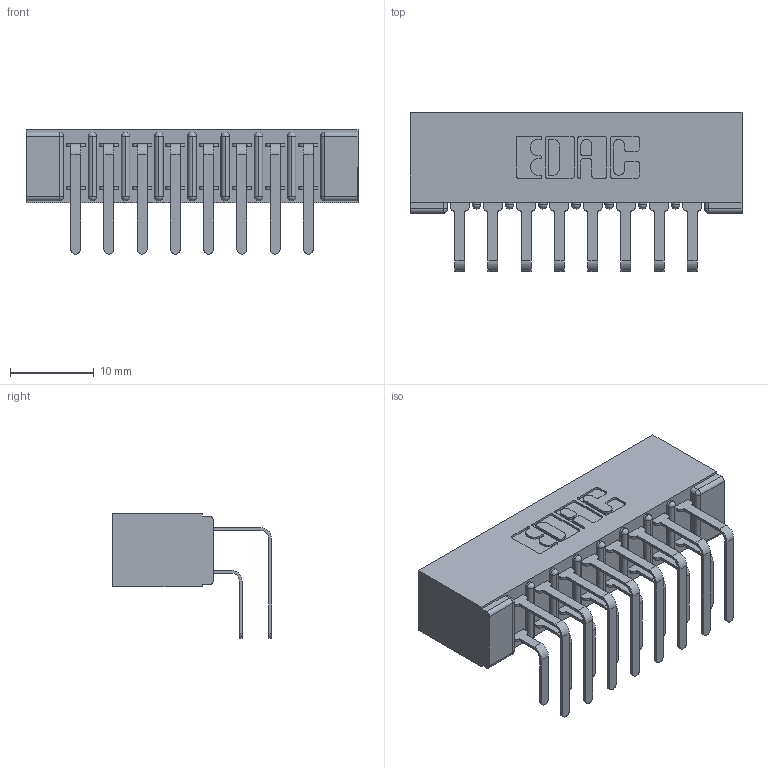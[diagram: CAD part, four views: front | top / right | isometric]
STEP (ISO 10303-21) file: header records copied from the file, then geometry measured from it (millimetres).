
FILE_DESCRIPTION (( 'STEP AP203' ), '1' );
FILE_NAME ('357-016-558-201.STEP', '2019-09-17T19:24:39', ( '' ), ( '' ), 'SwSTEP 2.0', 'SolidWorks 2016', '' );
FILE_SCHEMA (( 'CONFIG_CONTROL_DESIGN' ));
Length unit declared in the file: inch
Products named in the file (4): 357-016-558-201; 307-290-001_558 - 2 (Single); 307 Part_No Mounting Lugs; 307-290-001_558 559 - 1 (Single)
Assembly tree (17 placements, depth 2):
  357-016-558-201
    307 Part_No Mounting Lugs
    307-290-001_558 559 - 1 (Single)  x8
    307-290-001_558 - 2 (Single)  x8
Bounding box: 39.57 x 18.96 x 14.81 mm (x, y, z)
Volume: 2894.1 mm3; surface area: 5251.6 mm2
Topology: 17 solids, 17 shells, 919 faces, 2571 edges, 1666 vertices
Faces by surface type: plane 594, cylinder 307, sphere 18
Entity records: 12475 total; most frequent: CARTESIAN_POINT 2050, ORIENTED_EDGE 2026, DIRECTION 2021, EDGE_CURVE 1013, VECTOR 763, LINE 763, VERTEX_POINT 658, AXIS2_PLACEMENT_3D 629
